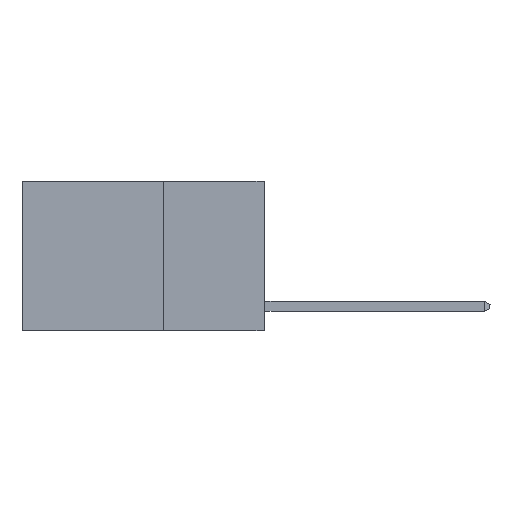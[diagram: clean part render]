
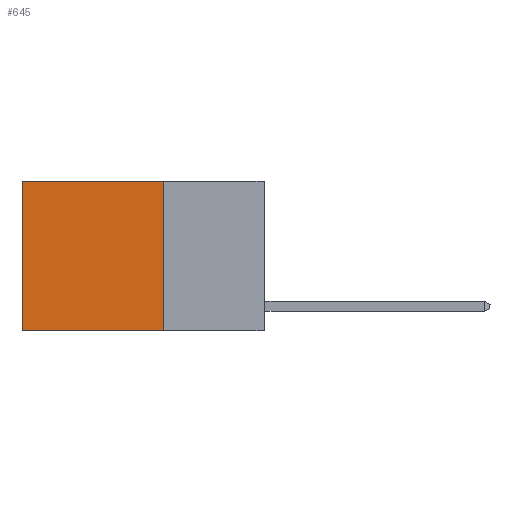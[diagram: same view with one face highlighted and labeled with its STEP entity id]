
A CAD part, left-side view. The second image highlights one B-rep face of the part: STEP entity #645.
In plain terms, the highlighted planar face has unit normal (-1, 0, 0).
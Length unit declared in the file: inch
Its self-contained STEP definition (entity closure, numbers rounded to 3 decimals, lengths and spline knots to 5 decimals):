
#645 = ADVANCED_FACE ( 'NONE', ( #13818 ), #17420, .F. ) ;
#2417 = CARTESIAN_POINT ( 'NONE',  ( 0.2625, 0.25, 0. ) ) ;
#3671 = CARTESIAN_POINT ( 'NONE',  ( 0.2625, 0.25, 0. ) ) ;
#4078 = DIRECTION ( 'NONE',  ( 1., 0., 0. ) ) ;
#5305 = ORIENTED_EDGE ( 'NONE', *, *, #6212, .F. ) ;
#5330 = DIRECTION ( 'NONE',  ( 0., 0., -1. ) ) ;
#5473 = LINE ( 'NONE', #9050, #17398 ) ;
#6212 = EDGE_CURVE ( 'NONE', #10312, #8180, #13806, .T. ) ;
#6584 = EDGE_CURVE ( 'NONE', #13736, #14044, #5473, .T. ) ;
#7184 = CARTESIAN_POINT ( 'NONE',  ( 0.2625, 0.6, 0. ) ) ;
#7813 = CARTESIAN_POINT ( 'NONE',  ( 0.2625, 0.6, -0.37 ) ) ;
#8153 = DIRECTION ( 'NONE',  ( 0., 0., -1. ) ) ;
#8180 = VERTEX_POINT ( 'NONE', #7813 ) ;
#8836 = EDGE_LOOP ( 'NONE', ( #18520, #5305, #14075, #20252 ) ) ;
#9050 = CARTESIAN_POINT ( 'NONE',  ( 0.2625, 0.25, 0. ) ) ;
#10088 = DIRECTION ( 'NONE',  ( 0., 0., -1. ) ) ;
#10198 = CARTESIAN_POINT ( 'NONE',  ( 0.2625, 0.25, 0. ) ) ;
#10312 = VERTEX_POINT ( 'NONE', #13003 ) ;
#10323 = EDGE_CURVE ( 'NONE', #14044, #8180, #19705, .T. ) ;
#10737 = AXIS2_PLACEMENT_3D ( 'NONE', #2417, #4078, #8153 ) ;
#13003 = CARTESIAN_POINT ( 'NONE',  ( 0.2625, 0.25, -0.37 ) ) ;
#13736 = VERTEX_POINT ( 'NONE', #3671 ) ;
#13769 = DIRECTION ( 'NONE',  ( 0., 1., 0. ) ) ;
#13806 = LINE ( 'NONE', #18200, #18414 ) ;
#13818 = FACE_OUTER_BOUND ( 'NONE', #8836, .T. ) ;
#14044 = VERTEX_POINT ( 'NONE', #7184 ) ;
#14075 = ORIENTED_EDGE ( 'NONE', *, *, #17617, .F. ) ;
#14701 = CARTESIAN_POINT ( 'NONE',  ( 0.2625, 0.6, 0. ) ) ;
#15231 = LINE ( 'NONE', #10198, #18140 ) ;
#16705 = DIRECTION ( 'NONE',  ( 0., 1., 0. ) ) ;
#17398 = VECTOR ( 'NONE', #13769, 39.37008 ) ;
#17420 = PLANE ( 'NONE',  #10737 ) ;
#17617 = EDGE_CURVE ( 'NONE', #13736, #10312, #15231, .T. ) ;
#18140 = VECTOR ( 'NONE', #5330, 39.37008 ) ;
#18200 = CARTESIAN_POINT ( 'NONE',  ( 0.2625, 0.25, -0.37 ) ) ;
#18414 = VECTOR ( 'NONE', #16705, 39.37008 ) ;
#18520 = ORIENTED_EDGE ( 'NONE', *, *, #10323, .T. ) ;
#19705 = LINE ( 'NONE', #14701, #20205 ) ;
#20205 = VECTOR ( 'NONE', #10088, 39.37008 ) ;
#20252 = ORIENTED_EDGE ( 'NONE', *, *, #6584, .T. ) ;
